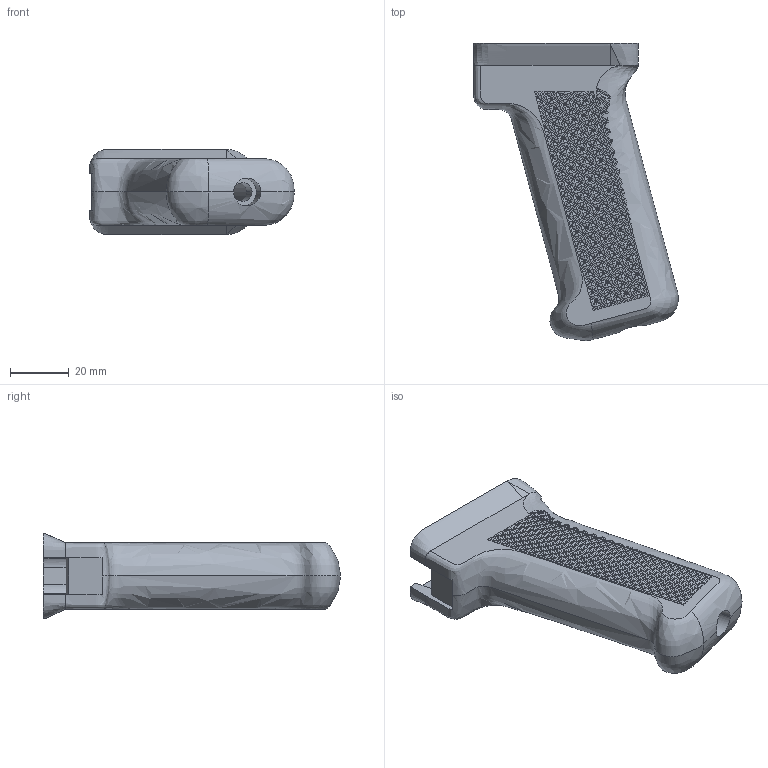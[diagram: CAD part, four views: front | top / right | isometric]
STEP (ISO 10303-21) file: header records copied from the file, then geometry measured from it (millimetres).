
FILE_DESCRIPTION (( 'STEP AP214' ), '1' );
FILE_NAME ('grip.STEP', '2015-01-19T02:49:01', ( 'eric' ), ( '' ), 'SwSTEP 2.0', 'SolidWorks 2012', '' );
FILE_SCHEMA (( 'AUTOMOTIVE_DESIGN' ));
Length unit declared in the file: millimetre
Products named in the file (1): grip
Bounding box: 69.69 x 101.24 x 29 mm (x, y, z)
Volume: 44025.7 mm3; surface area: 24137.2 mm2
Topology: 1 solids, 1 shells, 2247 faces, 4743 edges, 3040 vertices
Faces by surface type: plane 2206, bspline 27, cylinder 14
Entity records: 75086 total; most frequent: CARTESIAN_POINT 27259, ORIENTED_EDGE 9482, DIRECTION 8993, EDGE_CURVE 4741, LINE 4445, VECTOR 4445, VERTEX_POINT 3040, EDGE_LOOP 2793
